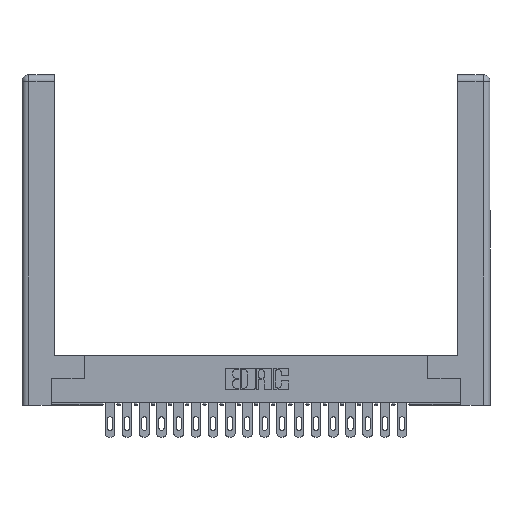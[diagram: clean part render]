
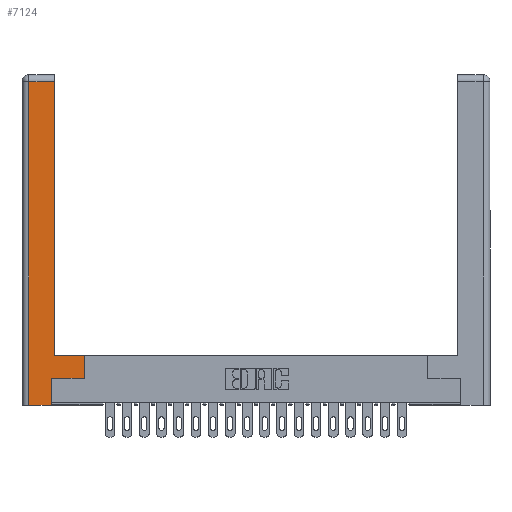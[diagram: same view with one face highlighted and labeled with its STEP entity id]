
A CAD part, top view. The second image highlights one B-rep face of the part: STEP entity #7124.
In plain terms, the highlighted planar face has unit normal (0, 0, 1).
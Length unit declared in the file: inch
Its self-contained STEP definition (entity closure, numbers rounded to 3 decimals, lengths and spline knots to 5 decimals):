
#33 = CARTESIAN_POINT ( 'NONE',  ( 0.0615, 2.94, 0. ) ) ;
#715 = ORIENTED_EDGE ( 'NONE', *, *, #11064, .T. ) ;
#730 = DIRECTION ( 'NONE',  ( 0., 1., 0. ) ) ;
#735 = PLANE ( 'NONE',  #3077 ) ;
#762 = CARTESIAN_POINT ( 'NONE',  ( 0.565, 0.45, 0. ) ) ;
#831 = EDGE_CURVE ( 'NONE', #5651, #7106, #3425, .T. ) ;
#1107 = ORIENTED_EDGE ( 'NONE', *, *, #6882, .T. ) ;
#1725 = VECTOR ( 'NONE', #18140, 39.37008 ) ;
#1995 = VECTOR ( 'NONE', #9726, 39.37008 ) ;
#2339 = CARTESIAN_POINT ( 'NONE',  ( 0., 0., 0. ) ) ;
#2956 = CARTESIAN_POINT ( 'NONE',  ( 0.265, 0., 0. ) ) ;
#2988 = CARTESIAN_POINT ( 'NONE',  ( 0.0615, 0., 0. ) ) ;
#3077 = AXIS2_PLACEMENT_3D ( 'NONE', #2339, #17847, #12810 ) ;
#3425 = LINE ( 'NONE', #21002, #17476 ) ;
#3576 = ORIENTED_EDGE ( 'NONE', *, *, #22179, .T. ) ;
#3869 = CARTESIAN_POINT ( 'NONE',  ( 0.565, 0.45, 0. ) ) ;
#4198 = CARTESIAN_POINT ( 'NONE',  ( 0.0615, 2.94, 0. ) ) ;
#4419 = CARTESIAN_POINT ( 'NONE',  ( 0.295, 3., 0. ) ) ;
#4607 = VECTOR ( 'NONE', #5547, 39.37008 ) ;
#4653 = VECTOR ( 'NONE', #12096, 39.37008 ) ;
#5099 = CARTESIAN_POINT ( 'NONE',  ( 0.265, 0.245, 0. ) ) ;
#5547 = DIRECTION ( 'NONE',  ( 0., 1., 0. ) ) ;
#5651 = VERTEX_POINT ( 'NONE', #3869 ) ;
#5704 = DIRECTION ( 'NONE',  ( 0., 1., 0. ) ) ;
#5747 = LINE ( 'NONE', #16317, #1725 ) ;
#5797 = FACE_OUTER_BOUND ( 'NONE', #18106, .T. ) ;
#6085 = VERTEX_POINT ( 'NONE', #2988 ) ;
#6113 = VERTEX_POINT ( 'NONE', #22623 ) ;
#6640 = CARTESIAN_POINT ( 'NONE',  ( 0.565, 0.245, 0. ) ) ;
#6860 = LINE ( 'NONE', #6640, #10849 ) ;
#6874 = ORIENTED_EDGE ( 'NONE', *, *, #831, .T. ) ;
#6882 = EDGE_CURVE ( 'NONE', #6113, #5651, #9598, .T. ) ;
#7106 = VERTEX_POINT ( 'NONE', #9122 ) ;
#7124 = ADVANCED_FACE ( 'NONE', ( #5797 ), #735, .F. ) ;
#7781 = ORIENTED_EDGE ( 'NONE', *, *, #17881, .T. ) ;
#8030 = EDGE_CURVE ( 'NONE', #10781, #8876, #10353, .T. ) ;
#8579 = CARTESIAN_POINT ( 'NONE',  ( 0.265, 0.245, 0. ) ) ;
#8833 = EDGE_CURVE ( 'NONE', #8876, #6113, #6860, .T. ) ;
#8876 = VERTEX_POINT ( 'NONE', #8579 ) ;
#9122 = CARTESIAN_POINT ( 'NONE',  ( 0.295, 0.45, 0. ) ) ;
#9279 = EDGE_CURVE ( 'NONE', #19232, #11853, #21285, .T. ) ;
#9598 = LINE ( 'NONE', #762, #20304 ) ;
#9726 = DIRECTION ( 'NONE',  ( 1., 0., 0. ) ) ;
#10353 = LINE ( 'NONE', #5099, #4607 ) ;
#10418 = DIRECTION ( 'NONE',  ( -1., 0., 0. ) ) ;
#10781 = VERTEX_POINT ( 'NONE', #22511 ) ;
#10849 = VECTOR ( 'NONE', #12151, 39.37008 ) ;
#11064 = EDGE_CURVE ( 'NONE', #11853, #6085, #5747, .T. ) ;
#11853 = VERTEX_POINT ( 'NONE', #4198 ) ;
#12096 = DIRECTION ( 'NONE',  ( -1., 0., 0. ) ) ;
#12151 = DIRECTION ( 'NONE',  ( 1., 0., 0. ) ) ;
#12810 = DIRECTION ( 'NONE',  ( -1., 0., 0. ) ) ;
#15871 = LINE ( 'NONE', #2956, #1995 ) ;
#16317 = CARTESIAN_POINT ( 'NONE',  ( 0.0615, 0., 0. ) ) ;
#16475 = LINE ( 'NONE', #4419, #17511 ) ;
#17043 = ORIENTED_EDGE ( 'NONE', *, *, #9279, .T. ) ;
#17204 = CARTESIAN_POINT ( 'NONE',  ( 0.295, 2.94, 0. ) ) ;
#17476 = VECTOR ( 'NONE', #10418, 39.37008 ) ;
#17511 = VECTOR ( 'NONE', #730, 39.37008 ) ;
#17847 = DIRECTION ( 'NONE',  ( 0., 0., -1. ) ) ;
#17881 = EDGE_CURVE ( 'NONE', #6085, #10781, #15871, .T. ) ;
#18106 = EDGE_LOOP ( 'NONE', ( #3576, #17043, #715, #7781, #18479, #19783, #1107, #6874 ) ) ;
#18140 = DIRECTION ( 'NONE',  ( 0., -1., 0. ) ) ;
#18479 = ORIENTED_EDGE ( 'NONE', *, *, #8030, .T. ) ;
#19232 = VERTEX_POINT ( 'NONE', #17204 ) ;
#19783 = ORIENTED_EDGE ( 'NONE', *, *, #8833, .T. ) ;
#20304 = VECTOR ( 'NONE', #5704, 39.37008 ) ;
#21002 = CARTESIAN_POINT ( 'NONE',  ( 0.295, 0.45, 0. ) ) ;
#21285 = LINE ( 'NONE', #33, #4653 ) ;
#22179 = EDGE_CURVE ( 'NONE', #7106, #19232, #16475, .T. ) ;
#22511 = CARTESIAN_POINT ( 'NONE',  ( 0.265, 0., 0. ) ) ;
#22623 = CARTESIAN_POINT ( 'NONE',  ( 0.565, 0.245, 0. ) ) ;
